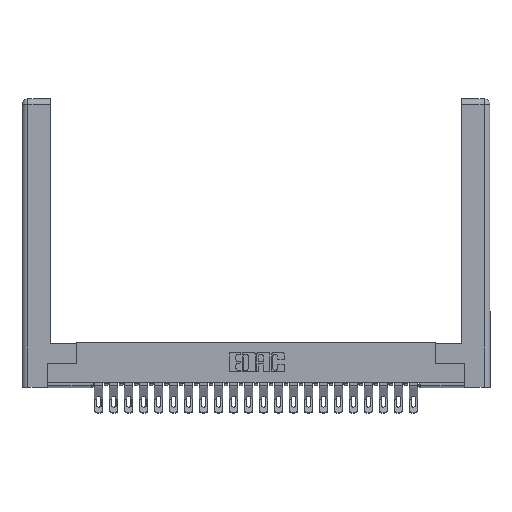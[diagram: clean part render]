
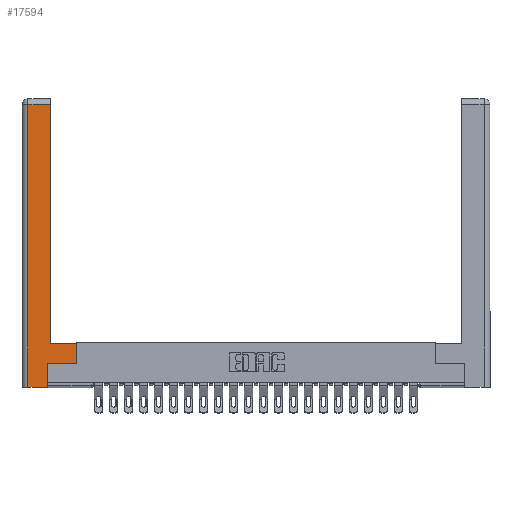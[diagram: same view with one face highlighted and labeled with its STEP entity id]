
A CAD part, top view. The second image highlights one B-rep face of the part: STEP entity #17594.
In plain terms, the highlighted planar face has unit normal (0, 0, 1).
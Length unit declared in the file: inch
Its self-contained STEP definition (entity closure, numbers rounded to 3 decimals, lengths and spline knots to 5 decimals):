
#847 = EDGE_CURVE ( 'NONE', #24085, #22357, #6040, .T. ) ;
#1472 = DIRECTION ( 'NONE',  ( 0., 0., -1. ) ) ;
#1903 = CARTESIAN_POINT ( 'NONE',  ( 0.565, 0.45, 0. ) ) ;
#2371 = VECTOR ( 'NONE', #17771, 39.37008 ) ;
#3054 = VECTOR ( 'NONE', #16929, 39.37008 ) ;
#3470 = VERTEX_POINT ( 'NONE', #20354 ) ;
#3542 = ORIENTED_EDGE ( 'NONE', *, *, #7972, .T. ) ;
#4733 = DIRECTION ( 'NONE',  ( 1., 0., 0. ) ) ;
#5061 = VERTEX_POINT ( 'NONE', #19203 ) ;
#5376 = ORIENTED_EDGE ( 'NONE', *, *, #7226, .T. ) ;
#6040 = LINE ( 'NONE', #16587, #15787 ) ;
#7002 = EDGE_CURVE ( 'NONE', #16671, #10964, #16952, .T. ) ;
#7226 = EDGE_CURVE ( 'NONE', #17098, #24085, #16926, .T. ) ;
#7303 = CARTESIAN_POINT ( 'NONE',  ( 0.265, 0.245, 0. ) ) ;
#7392 = LINE ( 'NONE', #8795, #11319 ) ;
#7546 = DIRECTION ( 'NONE',  ( -1., 0., 0. ) ) ;
#7972 = EDGE_CURVE ( 'NONE', #21351, #5061, #24154, .T. ) ;
#8265 = CARTESIAN_POINT ( 'NONE',  ( 0.295, 2.94, 0. ) ) ;
#8319 = CARTESIAN_POINT ( 'NONE',  ( 0.0615, 0., 0. ) ) ;
#8795 = CARTESIAN_POINT ( 'NONE',  ( 0.295, 3., 0. ) ) ;
#9257 = VECTOR ( 'NONE', #4733, 39.37008 ) ;
#9540 = CARTESIAN_POINT ( 'NONE',  ( 0.0615, 2.94, 0. ) ) ;
#9562 = DIRECTION ( 'NONE',  ( 1., 0., 0. ) ) ;
#9823 = EDGE_CURVE ( 'NONE', #5061, #3470, #20110, .T. ) ;
#10964 = VERTEX_POINT ( 'NONE', #14471 ) ;
#10966 = AXIS2_PLACEMENT_3D ( 'NONE', #17251, #1472, #7546 ) ;
#11244 = CARTESIAN_POINT ( 'NONE',  ( 0.565, 0.245, 0. ) ) ;
#11319 = VECTOR ( 'NONE', #14583, 39.37008 ) ;
#11394 = EDGE_CURVE ( 'NONE', #10964, #21351, #14257, .T. ) ;
#11893 = EDGE_CURVE ( 'NONE', #3470, #17098, #15455, .T. ) ;
#12530 = FACE_OUTER_BOUND ( 'NONE', #17159, .T. ) ;
#13098 = CARTESIAN_POINT ( 'NONE',  ( 0.565, 0.245, 0. ) ) ;
#13169 = PLANE ( 'NONE',  #10966 ) ;
#14257 = LINE ( 'NONE', #8319, #2371 ) ;
#14471 = CARTESIAN_POINT ( 'NONE',  ( 0.0615, 2.94, 0. ) ) ;
#14583 = DIRECTION ( 'NONE',  ( 0., 1., 0. ) ) ;
#14782 = VECTOR ( 'NONE', #19897, 39.37008 ) ;
#15455 = LINE ( 'NONE', #11244, #23956 ) ;
#15787 = VECTOR ( 'NONE', #22006, 39.37008 ) ;
#16005 = CARTESIAN_POINT ( 'NONE',  ( 0.565, 0.45, 0. ) ) ;
#16061 = CARTESIAN_POINT ( 'NONE',  ( 0.265, 0., 0. ) ) ;
#16587 = CARTESIAN_POINT ( 'NONE',  ( 0.295, 0.45, 0. ) ) ;
#16671 = VERTEX_POINT ( 'NONE', #8265 ) ;
#16926 = LINE ( 'NONE', #16005, #14782 ) ;
#16929 = DIRECTION ( 'NONE',  ( 0., 1., 0. ) ) ;
#16952 = LINE ( 'NONE', #9540, #17548 ) ;
#17098 = VERTEX_POINT ( 'NONE', #13098 ) ;
#17159 = EDGE_LOOP ( 'NONE', ( #24105, #19056, #24405, #3542, #19639, #22922, #5376, #24686 ) ) ;
#17251 = CARTESIAN_POINT ( 'NONE',  ( 0., 0., 0. ) ) ;
#17548 = VECTOR ( 'NONE', #19311, 39.37008 ) ;
#17594 = ADVANCED_FACE ( 'NONE', ( #12530 ), #13169, .F. ) ;
#17771 = DIRECTION ( 'NONE',  ( 0., -1., 0. ) ) ;
#19056 = ORIENTED_EDGE ( 'NONE', *, *, #7002, .T. ) ;
#19203 = CARTESIAN_POINT ( 'NONE',  ( 0.265, 0., 0. ) ) ;
#19311 = DIRECTION ( 'NONE',  ( -1., 0., 0. ) ) ;
#19639 = ORIENTED_EDGE ( 'NONE', *, *, #9823, .T. ) ;
#19897 = DIRECTION ( 'NONE',  ( 0., 1., 0. ) ) ;
#20110 = LINE ( 'NONE', #7303, #3054 ) ;
#20354 = CARTESIAN_POINT ( 'NONE',  ( 0.265, 0.245, 0. ) ) ;
#20483 = CARTESIAN_POINT ( 'NONE',  ( 0.295, 0.45, 0. ) ) ;
#21351 = VERTEX_POINT ( 'NONE', #23070 ) ;
#22006 = DIRECTION ( 'NONE',  ( -1., 0., 0. ) ) ;
#22357 = VERTEX_POINT ( 'NONE', #20483 ) ;
#22922 = ORIENTED_EDGE ( 'NONE', *, *, #11893, .T. ) ;
#23070 = CARTESIAN_POINT ( 'NONE',  ( 0.0615, 0., 0. ) ) ;
#23956 = VECTOR ( 'NONE', #9562, 39.37008 ) ;
#24085 = VERTEX_POINT ( 'NONE', #1903 ) ;
#24105 = ORIENTED_EDGE ( 'NONE', *, *, #24378, .T. ) ;
#24154 = LINE ( 'NONE', #16061, #9257 ) ;
#24378 = EDGE_CURVE ( 'NONE', #22357, #16671, #7392, .T. ) ;
#24405 = ORIENTED_EDGE ( 'NONE', *, *, #11394, .T. ) ;
#24686 = ORIENTED_EDGE ( 'NONE', *, *, #847, .T. ) ;
